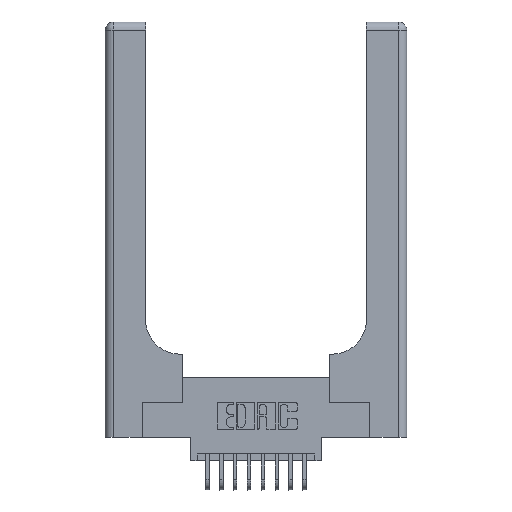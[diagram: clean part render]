
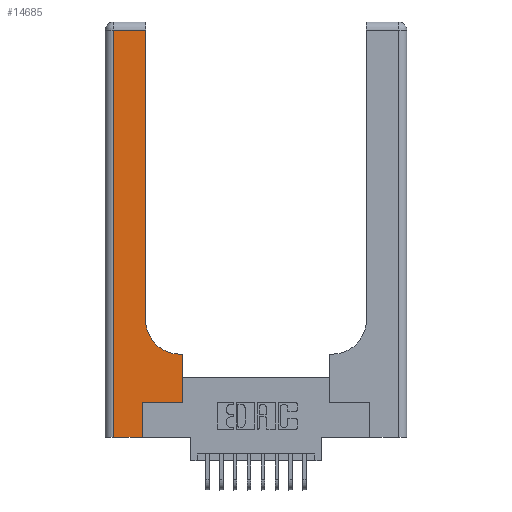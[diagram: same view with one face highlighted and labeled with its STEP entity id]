
A CAD part, top view. The second image highlights one B-rep face of the part: STEP entity #14685.
In plain terms, the highlighted planar face has unit normal (0, 0, 1).
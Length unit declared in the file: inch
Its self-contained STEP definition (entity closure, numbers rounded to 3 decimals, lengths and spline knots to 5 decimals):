
#10 = VERTEX_POINT ( 'NONE', #9947 ) ;
#160 = DIRECTION ( 'NONE',  ( 0., 1., 0. ) ) ;
#355 = VECTOR ( 'NONE', #3369, 39.37008 ) ;
#405 = VECTOR ( 'NONE', #3947, 39.37008 ) ;
#615 = VERTEX_POINT ( 'NONE', #8385 ) ;
#849 = DIRECTION ( 'NONE',  ( -1., 0., 0. ) ) ;
#912 = VECTOR ( 'NONE', #11999, 39.37008 ) ;
#1209 = DIRECTION ( 'NONE',  ( 1., 0., 0. ) ) ;
#1277 = VERTEX_POINT ( 'NONE', #11402 ) ;
#1345 = CARTESIAN_POINT ( 'NONE',  ( 0.5415, 0.85, 0.37 ) ) ;
#1641 = LINE ( 'NONE', #6161, #355 ) ;
#1768 = ORIENTED_EDGE ( 'NONE', *, *, #11415, .T. ) ;
#1860 = ORIENTED_EDGE ( 'NONE', *, *, #16201, .T. ) ;
#1980 = FACE_OUTER_BOUND ( 'NONE', #14966, .T. ) ;
#2196 = AXIS2_PLACEMENT_3D ( 'NONE', #13049, #9011, #849 ) ;
#2413 = VECTOR ( 'NONE', #7211, 39.37008 ) ;
#2493 = ORIENTED_EDGE ( 'NONE', *, *, #10444, .T. ) ;
#2506 = DIRECTION ( 'NONE',  ( 0., -1., 0. ) ) ;
#2843 = CARTESIAN_POINT ( 'NONE',  ( 0.06, 2.94, 0.37 ) ) ;
#3369 = DIRECTION ( 'NONE',  ( -1., 0., 0. ) ) ;
#3924 = LINE ( 'NONE', #5391, #7811 ) ;
#3947 = DIRECTION ( 'NONE',  ( 0., 1., 0. ) ) ;
#4134 = DIRECTION ( 'NONE',  ( 0., 0., -1. ) ) ;
#4376 = CARTESIAN_POINT ( 'NONE',  ( 0.269, 0.25, 0.37 ) ) ;
#5351 = VERTEX_POINT ( 'NONE', #10974 ) ;
#5391 = CARTESIAN_POINT ( 'NONE',  ( 0., 0., 0.37 ) ) ;
#5639 = CIRCLE ( 'NONE', #14554, 0.25 ) ;
#6161 = CARTESIAN_POINT ( 'NONE',  ( 0., 2.94, 0.37 ) ) ;
#6395 = ORIENTED_EDGE ( 'NONE', *, *, #17048, .T. ) ;
#6551 = LINE ( 'NONE', #4376, #2413 ) ;
#6893 = EDGE_CURVE ( 'NONE', #1277, #615, #7406, .T. ) ;
#6907 = LINE ( 'NONE', #12165, #405 ) ;
#7006 = VERTEX_POINT ( 'NONE', #17811 ) ;
#7130 = LINE ( 'NONE', #10278, #15702 ) ;
#7145 = EDGE_CURVE ( 'NONE', #615, #7006, #6551, .T. ) ;
#7159 = CARTESIAN_POINT ( 'NONE',  ( 0.5585, 0.25, 0.37 ) ) ;
#7211 = DIRECTION ( 'NONE',  ( 1., 0., 0. ) ) ;
#7310 = ORIENTED_EDGE ( 'NONE', *, *, #17738, .T. ) ;
#7406 = LINE ( 'NONE', #9321, #912 ) ;
#7543 = EDGE_CURVE ( 'NONE', #17828, #1277, #3924, .T. ) ;
#7706 = CARTESIAN_POINT ( 'NONE',  ( 0.2915, 0.6, 0.37 ) ) ;
#7811 = VECTOR ( 'NONE', #1209, 39.37008 ) ;
#8385 = CARTESIAN_POINT ( 'NONE',  ( 0.269, 0.25, 0.37 ) ) ;
#9011 = DIRECTION ( 'NONE',  ( 0., 0., -1. ) ) ;
#9025 = DIRECTION ( 'NONE',  ( -1., 0., 0. ) ) ;
#9321 = CARTESIAN_POINT ( 'NONE',  ( 0.269, 0., 0.37 ) ) ;
#9947 = CARTESIAN_POINT ( 'NONE',  ( 0.5585, 0.6, 0.37 ) ) ;
#10278 = CARTESIAN_POINT ( 'NONE',  ( 0.06, 3., 0.37 ) ) ;
#10444 = EDGE_CURVE ( 'NONE', #17800, #10747, #1641, .T. ) ;
#10661 = LINE ( 'NONE', #7159, #12590 ) ;
#10747 = VERTEX_POINT ( 'NONE', #2843 ) ;
#10974 = CARTESIAN_POINT ( 'NONE',  ( 0.5415, 0.6, 0.37 ) ) ;
#11402 = CARTESIAN_POINT ( 'NONE',  ( 0.269, 0., 0.37 ) ) ;
#11415 = EDGE_CURVE ( 'NONE', #7006, #10, #10661, .T. ) ;
#11999 = DIRECTION ( 'NONE',  ( 0., 1., 0. ) ) ;
#12165 = CARTESIAN_POINT ( 'NONE',  ( 0.2915, 3., 0.37 ) ) ;
#12590 = VECTOR ( 'NONE', #160, 39.37008 ) ;
#12636 = ORIENTED_EDGE ( 'NONE', *, *, #6893, .T. ) ;
#12719 = ORIENTED_EDGE ( 'NONE', *, *, #7145, .T. ) ;
#13049 = CARTESIAN_POINT ( 'NONE',  ( 0., 3., 0.37 ) ) ;
#13522 = EDGE_CURVE ( 'NONE', #10, #5351, #17089, .T. ) ;
#13587 = CARTESIAN_POINT ( 'NONE',  ( 0.06, 0., 0.37 ) ) ;
#13721 = DIRECTION ( 'NONE',  ( 1., 0., 0. ) ) ;
#14190 = ORIENTED_EDGE ( 'NONE', *, *, #7543, .T. ) ;
#14304 = VECTOR ( 'NONE', #9025, 39.37008 ) ;
#14508 = PLANE ( 'NONE',  #2196 ) ;
#14554 = AXIS2_PLACEMENT_3D ( 'NONE', #1345, #4134, #13721 ) ;
#14685 = ADVANCED_FACE ( 'NONE', ( #1980 ), #14508, .F. ) ;
#14888 = ORIENTED_EDGE ( 'NONE', *, *, #13522, .T. ) ;
#14966 = EDGE_LOOP ( 'NONE', ( #7310, #2493, #6395, #14190, #12636, #12719, #1768, #14888, #1860 ) ) ;
#15702 = VECTOR ( 'NONE', #2506, 39.37008 ) ;
#16074 = CARTESIAN_POINT ( 'NONE',  ( 0.2915, 2.94, 0.37 ) ) ;
#16201 = EDGE_CURVE ( 'NONE', #5351, #16397, #5639, .T. ) ;
#16397 = VERTEX_POINT ( 'NONE', #16859 ) ;
#16859 = CARTESIAN_POINT ( 'NONE',  ( 0.2915, 0.85, 0.37 ) ) ;
#17048 = EDGE_CURVE ( 'NONE', #10747, #17828, #7130, .T. ) ;
#17089 = LINE ( 'NONE', #7706, #14304 ) ;
#17738 = EDGE_CURVE ( 'NONE', #16397, #17800, #6907, .T. ) ;
#17800 = VERTEX_POINT ( 'NONE', #16074 ) ;
#17811 = CARTESIAN_POINT ( 'NONE',  ( 0.5585, 0.25, 0.37 ) ) ;
#17828 = VERTEX_POINT ( 'NONE', #13587 ) ;
